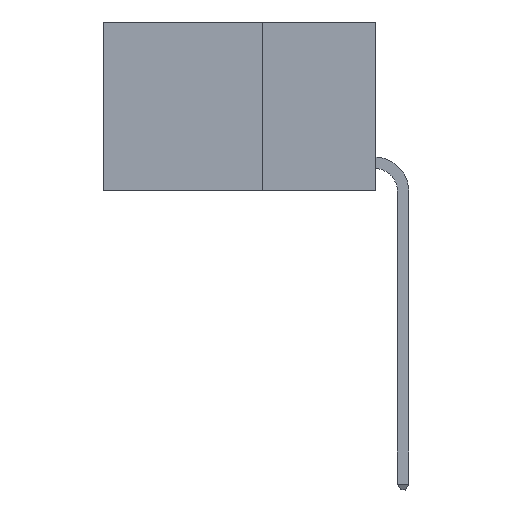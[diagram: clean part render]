
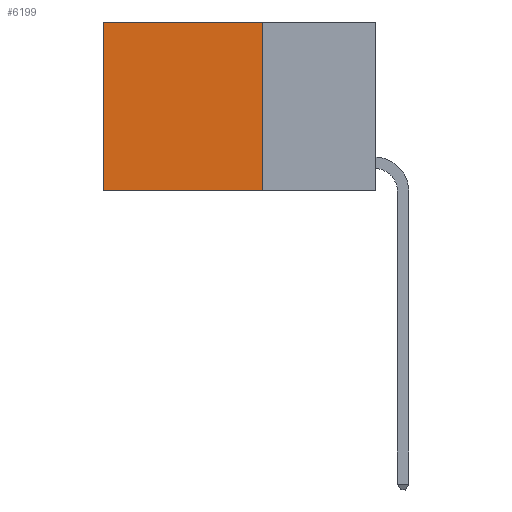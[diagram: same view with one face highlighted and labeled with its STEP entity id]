
A CAD part, left-side view. The second image highlights one B-rep face of the part: STEP entity #6199.
In plain terms, the highlighted planar face has unit normal (-1, 0, 0).
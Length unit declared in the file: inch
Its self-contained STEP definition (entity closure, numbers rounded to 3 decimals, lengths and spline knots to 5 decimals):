
#535 = LINE ( 'NONE', #11779, #2371 ) ;
#802 = LINE ( 'NONE', #5527, #11547 ) ;
#1203 = DIRECTION ( 'NONE',  ( 0., 0., -1. ) ) ;
#1302 = CARTESIAN_POINT ( 'NONE',  ( 0.2625, 0.25, 0. ) ) ;
#1726 = ORIENTED_EDGE ( 'NONE', *, *, #18464, .F. ) ;
#2281 = CARTESIAN_POINT ( 'NONE',  ( 0.2625, 0.25, 0. ) ) ;
#2371 = VECTOR ( 'NONE', #11887, 39.37008 ) ;
#3482 = VERTEX_POINT ( 'NONE', #18646 ) ;
#4669 = VERTEX_POINT ( 'NONE', #2281 ) ;
#4709 = CARTESIAN_POINT ( 'NONE',  ( 0.2625, 0.6, -0.37 ) ) ;
#4954 = LINE ( 'NONE', #19845, #9338 ) ;
#5527 = CARTESIAN_POINT ( 'NONE',  ( 0.2625, 0.6, 0. ) ) ;
#5628 = ORIENTED_EDGE ( 'NONE', *, *, #16614, .T. ) ;
#6199 = ADVANCED_FACE ( 'NONE', ( #17398 ), #12896, .F. ) ;
#8154 = DIRECTION ( 'NONE',  ( 0., 0., -1. ) ) ;
#8548 = CARTESIAN_POINT ( 'NONE',  ( 0.2625, 0.25, -0.37 ) ) ;
#9175 = LINE ( 'NONE', #1302, #19762 ) ;
#9338 = VECTOR ( 'NONE', #14808, 39.37008 ) ;
#11547 = VECTOR ( 'NONE', #15298, 39.37008 ) ;
#11779 = CARTESIAN_POINT ( 'NONE',  ( 0.2625, 0.25, 0. ) ) ;
#11887 = DIRECTION ( 'NONE',  ( 0., 1., 0. ) ) ;
#12896 = PLANE ( 'NONE',  #14290 ) ;
#12991 = EDGE_CURVE ( 'NONE', #16998, #16391, #4954, .T. ) ;
#14290 = AXIS2_PLACEMENT_3D ( 'NONE', #17509, #19285, #8154 ) ;
#14546 = EDGE_LOOP ( 'NONE', ( #5628, #18832, #1726, #16067 ) ) ;
#14808 = DIRECTION ( 'NONE',  ( 0., 1., 0. ) ) ;
#15298 = DIRECTION ( 'NONE',  ( 0., 0., -1. ) ) ;
#16067 = ORIENTED_EDGE ( 'NONE', *, *, #19133, .T. ) ;
#16391 = VERTEX_POINT ( 'NONE', #4709 ) ;
#16614 = EDGE_CURVE ( 'NONE', #3482, #16391, #802, .T. ) ;
#16998 = VERTEX_POINT ( 'NONE', #8548 ) ;
#17398 = FACE_OUTER_BOUND ( 'NONE', #14546, .T. ) ;
#17509 = CARTESIAN_POINT ( 'NONE',  ( 0.2625, 0.25, 0. ) ) ;
#18464 = EDGE_CURVE ( 'NONE', #4669, #16998, #9175, .T. ) ;
#18646 = CARTESIAN_POINT ( 'NONE',  ( 0.2625, 0.6, 0. ) ) ;
#18832 = ORIENTED_EDGE ( 'NONE', *, *, #12991, .F. ) ;
#19133 = EDGE_CURVE ( 'NONE', #4669, #3482, #535, .T. ) ;
#19285 = DIRECTION ( 'NONE',  ( 1., 0., 0. ) ) ;
#19762 = VECTOR ( 'NONE', #1203, 39.37008 ) ;
#19845 = CARTESIAN_POINT ( 'NONE',  ( 0.2625, 0.25, -0.37 ) ) ;
